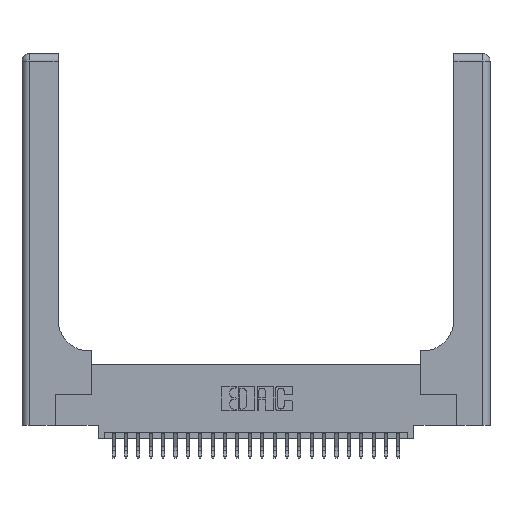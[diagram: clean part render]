
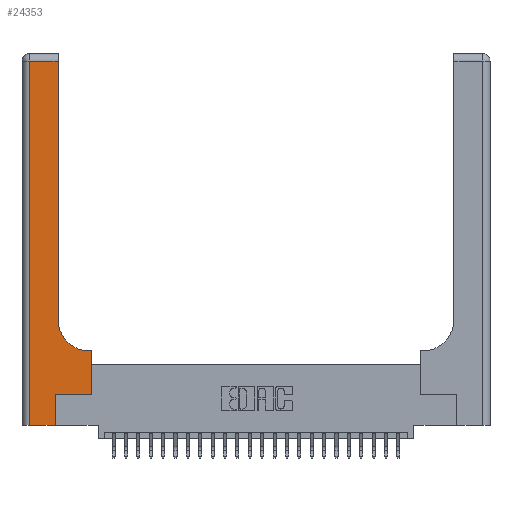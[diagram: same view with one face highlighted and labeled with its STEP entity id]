
A CAD part, top view. The second image highlights one B-rep face of the part: STEP entity #24353.
In plain terms, the highlighted planar face has unit normal (0, 0, 1).
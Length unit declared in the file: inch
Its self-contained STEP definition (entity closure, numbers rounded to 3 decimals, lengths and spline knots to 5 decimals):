
#271 = VERTEX_POINT ( 'NONE', #20487 ) ;
#317 = DIRECTION ( 'NONE',  ( 0., 0., -1. ) ) ;
#626 = LINE ( 'NONE', #5409, #22330 ) ;
#684 = VECTOR ( 'NONE', #21035, 39.37008 ) ;
#1132 = VECTOR ( 'NONE', #10897, 39.37008 ) ;
#1342 = AXIS2_PLACEMENT_3D ( 'NONE', #20785, #317, #14883 ) ;
#1469 = CARTESIAN_POINT ( 'NONE',  ( 0.5585, 0.6, 0.37 ) ) ;
#2033 = LINE ( 'NONE', #9212, #11476 ) ;
#2430 = ORIENTED_EDGE ( 'NONE', *, *, #10878, .T. ) ;
#2564 = CARTESIAN_POINT ( 'NONE',  ( 0.5585, 0.25, 0.37 ) ) ;
#3030 = DIRECTION ( 'NONE',  ( -1., 0., 0. ) ) ;
#3123 = CARTESIAN_POINT ( 'NONE',  ( 0.2915, 0.6, 0.37 ) ) ;
#3413 = ORIENTED_EDGE ( 'NONE', *, *, #26460, .T. ) ;
#3879 = EDGE_CURVE ( 'NONE', #24725, #7701, #2033, .T. ) ;
#4085 = ORIENTED_EDGE ( 'NONE', *, *, #6004, .T. ) ;
#4293 = CARTESIAN_POINT ( 'NONE',  ( 0.269, 0., 0.37 ) ) ;
#4800 = VERTEX_POINT ( 'NONE', #1469 ) ;
#4866 = CARTESIAN_POINT ( 'NONE',  ( 0.2915, 3., 0.37 ) ) ;
#5304 = DIRECTION ( 'NONE',  ( 1., 0., 0. ) ) ;
#5409 = CARTESIAN_POINT ( 'NONE',  ( 0., 0., 0.37 ) ) ;
#5696 = CARTESIAN_POINT ( 'NONE',  ( 0.269, 0.25, 0.37 ) ) ;
#6004 = EDGE_CURVE ( 'NONE', #271, #7348, #626, .T. ) ;
#6053 = VERTEX_POINT ( 'NONE', #12077 ) ;
#6163 = VECTOR ( 'NONE', #7424, 39.37008 ) ;
#6423 = VECTOR ( 'NONE', #9087, 39.37008 ) ;
#6833 = EDGE_CURVE ( 'NONE', #7701, #4800, #26056, .T. ) ;
#6854 = LINE ( 'NONE', #4866, #684 ) ;
#6983 = EDGE_CURVE ( 'NONE', #7348, #24725, #15426, .T. ) ;
#7020 = CARTESIAN_POINT ( 'NONE',  ( 0.5585, 0.25, 0.37 ) ) ;
#7050 = VERTEX_POINT ( 'NONE', #23365 ) ;
#7348 = VERTEX_POINT ( 'NONE', #19969 ) ;
#7424 = DIRECTION ( 'NONE',  ( 0., -1., 0. ) ) ;
#7701 = VERTEX_POINT ( 'NONE', #2564 ) ;
#7740 = CIRCLE ( 'NONE', #22968, 0.25 ) ;
#8418 = LINE ( 'NONE', #19900, #6163 ) ;
#9087 = DIRECTION ( 'NONE',  ( -1., 0., 0. ) ) ;
#9212 = CARTESIAN_POINT ( 'NONE',  ( 0.269, 0.25, 0.37 ) ) ;
#9654 = VECTOR ( 'NONE', #3030, 39.37008 ) ;
#10007 = EDGE_CURVE ( 'NONE', #14894, #271, #8418, .T. ) ;
#10846 = EDGE_CURVE ( 'NONE', #6053, #14894, #13271, .T. ) ;
#10878 = EDGE_CURVE ( 'NONE', #16167, #7050, #7740, .T. ) ;
#10897 = DIRECTION ( 'NONE',  ( 0., 1., 0. ) ) ;
#11476 = VECTOR ( 'NONE', #5304, 39.37008 ) ;
#12077 = CARTESIAN_POINT ( 'NONE',  ( 0.2915, 2.94, 0.37 ) ) ;
#12171 = VECTOR ( 'NONE', #21564, 39.37008 ) ;
#12190 = DIRECTION ( 'NONE',  ( 0., 0., -1. ) ) ;
#13271 = LINE ( 'NONE', #15574, #6423 ) ;
#14883 = DIRECTION ( 'NONE',  ( -1., 0., 0. ) ) ;
#14894 = VERTEX_POINT ( 'NONE', #26195 ) ;
#15426 = LINE ( 'NONE', #4293, #1132 ) ;
#15574 = CARTESIAN_POINT ( 'NONE',  ( 0., 2.94, 0.37 ) ) ;
#16167 = VERTEX_POINT ( 'NONE', #24079 ) ;
#17026 = PLANE ( 'NONE',  #1342 ) ;
#17269 = EDGE_CURVE ( 'NONE', #7050, #6053, #6854, .T. ) ;
#18025 = ORIENTED_EDGE ( 'NONE', *, *, #6833, .T. ) ;
#18203 = ORIENTED_EDGE ( 'NONE', *, *, #17269, .T. ) ;
#18653 = EDGE_LOOP ( 'NONE', ( #18203, #25403, #24898, #4085, #22237, #20227, #18025, #3413, #2430 ) ) ;
#19900 = CARTESIAN_POINT ( 'NONE',  ( 0.06, 3., 0.37 ) ) ;
#19969 = CARTESIAN_POINT ( 'NONE',  ( 0.269, 0., 0.37 ) ) ;
#20227 = ORIENTED_EDGE ( 'NONE', *, *, #3879, .T. ) ;
#20381 = DIRECTION ( 'NONE',  ( 1., 0., 0. ) ) ;
#20460 = CARTESIAN_POINT ( 'NONE',  ( 0.5415, 0.85, 0.37 ) ) ;
#20487 = CARTESIAN_POINT ( 'NONE',  ( 0.06, 0., 0.37 ) ) ;
#20785 = CARTESIAN_POINT ( 'NONE',  ( 0., 3., 0.37 ) ) ;
#21035 = DIRECTION ( 'NONE',  ( 0., 1., 0. ) ) ;
#21266 = LINE ( 'NONE', #3123, #9654 ) ;
#21369 = FACE_OUTER_BOUND ( 'NONE', #18653, .T. ) ;
#21564 = DIRECTION ( 'NONE',  ( 0., 1., 0. ) ) ;
#22237 = ORIENTED_EDGE ( 'NONE', *, *, #6983, .T. ) ;
#22330 = VECTOR ( 'NONE', #20381, 39.37008 ) ;
#22968 = AXIS2_PLACEMENT_3D ( 'NONE', #20460, #12190, #24646 ) ;
#23365 = CARTESIAN_POINT ( 'NONE',  ( 0.2915, 0.85, 0.37 ) ) ;
#24079 = CARTESIAN_POINT ( 'NONE',  ( 0.5415, 0.6, 0.37 ) ) ;
#24353 = ADVANCED_FACE ( 'NONE', ( #21369 ), #17026, .F. ) ;
#24646 = DIRECTION ( 'NONE',  ( 1., 0., 0. ) ) ;
#24725 = VERTEX_POINT ( 'NONE', #5696 ) ;
#24898 = ORIENTED_EDGE ( 'NONE', *, *, #10007, .T. ) ;
#25403 = ORIENTED_EDGE ( 'NONE', *, *, #10846, .T. ) ;
#26056 = LINE ( 'NONE', #7020, #12171 ) ;
#26195 = CARTESIAN_POINT ( 'NONE',  ( 0.06, 2.94, 0.37 ) ) ;
#26460 = EDGE_CURVE ( 'NONE', #4800, #16167, #21266, .T. ) ;
